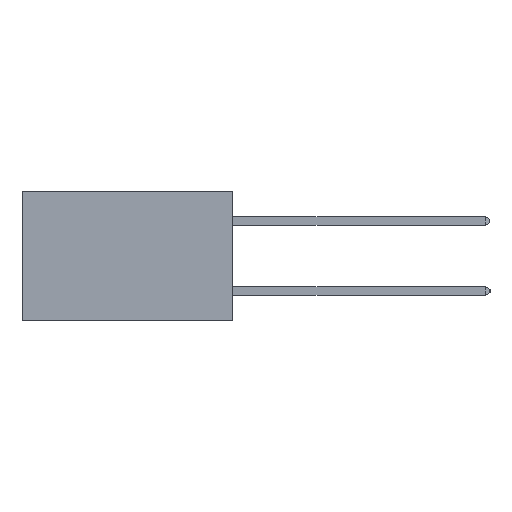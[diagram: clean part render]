
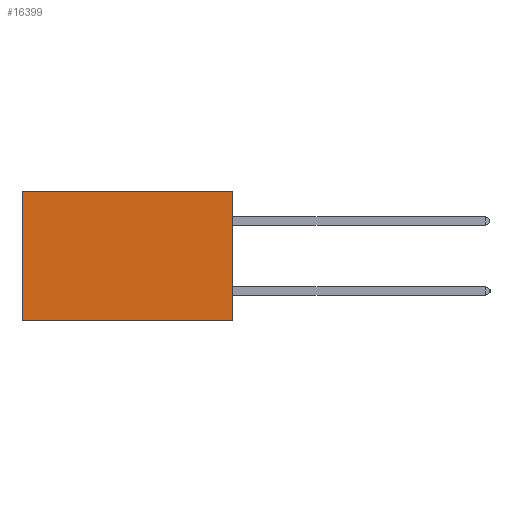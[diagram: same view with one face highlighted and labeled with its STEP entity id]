
A CAD part, left-side view. The second image highlights one B-rep face of the part: STEP entity #16399.
In plain terms, the highlighted planar face has unit normal (-1, 0, 0).
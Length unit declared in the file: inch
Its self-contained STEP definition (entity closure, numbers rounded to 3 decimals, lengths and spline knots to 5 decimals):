
#408 = VERTEX_POINT ( 'NONE', #20367 ) ;
#1424 = CARTESIAN_POINT ( 'NONE',  ( 0.2875, 0., 0. ) ) ;
#1823 = VECTOR ( 'NONE', #13451, 39.37008 ) ;
#2278 = VERTEX_POINT ( 'NONE', #7253 ) ;
#2889 = LINE ( 'NONE', #19920, #1823 ) ;
#3114 = DIRECTION ( 'NONE',  ( 0., 0., -1. ) ) ;
#4692 = LINE ( 'NONE', #8667, #17396 ) ;
#4911 = ORIENTED_EDGE ( 'NONE', *, *, #16603, .T. ) ;
#5206 = ORIENTED_EDGE ( 'NONE', *, *, #17192, .F. ) ;
#5464 = LINE ( 'NONE', #20382, #9922 ) ;
#5597 = EDGE_LOOP ( 'NONE', ( #15739, #10174, #5206, #4911 ) ) ;
#5940 = VERTEX_POINT ( 'NONE', #9755 ) ;
#6424 = PLANE ( 'NONE',  #14346 ) ;
#6736 = DIRECTION ( 'NONE',  ( 0., 0., -1. ) ) ;
#6779 = VECTOR ( 'NONE', #6736, 39.37008 ) ;
#7253 = CARTESIAN_POINT ( 'NONE',  ( 0.2875, 0.6, 0. ) ) ;
#8667 = CARTESIAN_POINT ( 'NONE',  ( 0.2875, 0., 0. ) ) ;
#8809 = EDGE_CURVE ( 'NONE', #5940, #408, #2889, .T. ) ;
#9755 = CARTESIAN_POINT ( 'NONE',  ( 0.2875, 0., -0.37 ) ) ;
#9922 = VECTOR ( 'NONE', #17080, 39.37008 ) ;
#10174 = ORIENTED_EDGE ( 'NONE', *, *, #8809, .F. ) ;
#13073 = DIRECTION ( 'NONE',  ( 1., 0., 0. ) ) ;
#13282 = FACE_OUTER_BOUND ( 'NONE', #5597, .T. ) ;
#13370 = CARTESIAN_POINT ( 'NONE',  ( 0.2875, 0.6, 0. ) ) ;
#13451 = DIRECTION ( 'NONE',  ( 0., 1., 0. ) ) ;
#14012 = CARTESIAN_POINT ( 'NONE',  ( 0.2875, 0., 0. ) ) ;
#14346 = AXIS2_PLACEMENT_3D ( 'NONE', #1424, #13073, #3114 ) ;
#15739 = ORIENTED_EDGE ( 'NONE', *, *, #20679, .T. ) ;
#16106 = VERTEX_POINT ( 'NONE', #14012 ) ;
#16399 = ADVANCED_FACE ( 'NONE', ( #13282 ), #6424, .F. ) ;
#16603 = EDGE_CURVE ( 'NONE', #16106, #2278, #4692, .T. ) ;
#16943 = DIRECTION ( 'NONE',  ( 0., 1., 0. ) ) ;
#17080 = DIRECTION ( 'NONE',  ( 0., 0., -1. ) ) ;
#17192 = EDGE_CURVE ( 'NONE', #16106, #5940, #5464, .T. ) ;
#17396 = VECTOR ( 'NONE', #16943, 39.37008 ) ;
#19918 = LINE ( 'NONE', #13370, #6779 ) ;
#19920 = CARTESIAN_POINT ( 'NONE',  ( 0.2875, 0., -0.37 ) ) ;
#20367 = CARTESIAN_POINT ( 'NONE',  ( 0.2875, 0.6, -0.37 ) ) ;
#20382 = CARTESIAN_POINT ( 'NONE',  ( 0.2875, 0., 0. ) ) ;
#20679 = EDGE_CURVE ( 'NONE', #2278, #408, #19918, .T. ) ;
